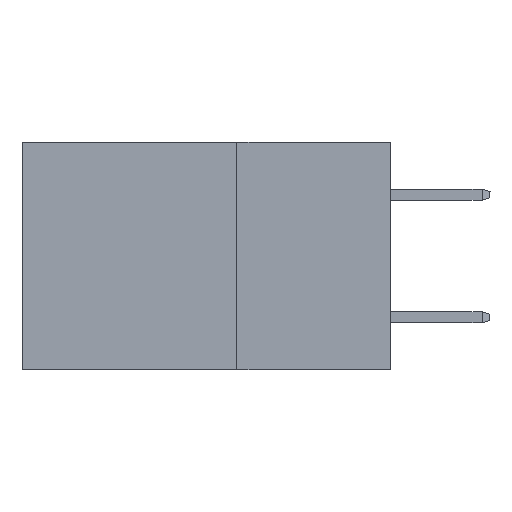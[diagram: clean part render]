
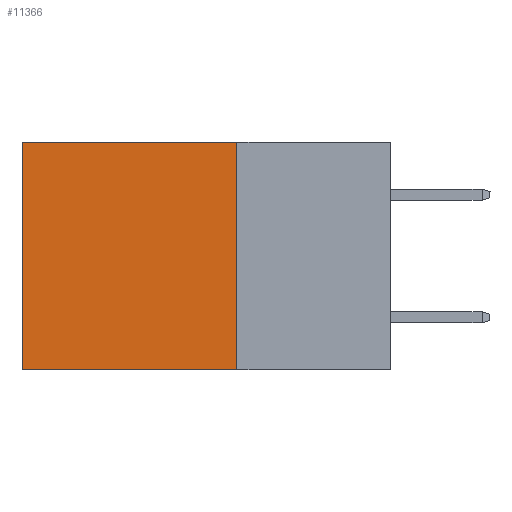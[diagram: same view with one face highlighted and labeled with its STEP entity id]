
A CAD part, left-side view. The second image highlights one B-rep face of the part: STEP entity #11366.
In plain terms, the highlighted planar face has unit normal (-1, 0, 0).
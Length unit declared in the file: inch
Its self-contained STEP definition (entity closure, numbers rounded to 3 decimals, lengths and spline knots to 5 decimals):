
#605 = CARTESIAN_POINT ( 'NONE',  ( 0.2875, 0.25, 0. ) ) ;
#1740 = VERTEX_POINT ( 'NONE', #13601 ) ;
#1962 = CARTESIAN_POINT ( 'NONE',  ( 0.2875, 0.25, 0. ) ) ;
#2853 = EDGE_CURVE ( 'NONE', #20786, #1740, #7967, .T. ) ;
#4057 = PLANE ( 'NONE',  #20959 ) ;
#6054 = ORIENTED_EDGE ( 'NONE', *, *, #20339, .T. ) ;
#6166 = VERTEX_POINT ( 'NONE', #6320 ) ;
#6305 = CARTESIAN_POINT ( 'NONE',  ( 0.2875, 0.25, 0. ) ) ;
#6320 = CARTESIAN_POINT ( 'NONE',  ( 0.2875, 0.25, -0.37 ) ) ;
#7039 = VECTOR ( 'NONE', #7184, 39.37008 ) ;
#7184 = DIRECTION ( 'NONE',  ( 0., 1., 0. ) ) ;
#7634 = DIRECTION ( 'NONE',  ( 1., 0., 0. ) ) ;
#7967 = LINE ( 'NONE', #13426, #21294 ) ;
#8365 = CARTESIAN_POINT ( 'NONE',  ( 0.2875, 0.6, 0. ) ) ;
#10256 = EDGE_CURVE ( 'NONE', #6166, #1740, #15493, .T. ) ;
#11265 = CARTESIAN_POINT ( 'NONE',  ( 0.2875, 0.25, -0.37 ) ) ;
#11366 = ADVANCED_FACE ( 'NONE', ( #20849 ), #4057, .F. ) ;
#11395 = VECTOR ( 'NONE', #18230, 39.37008 ) ;
#12250 = VERTEX_POINT ( 'NONE', #6305 ) ;
#12345 = ORIENTED_EDGE ( 'NONE', *, *, #10256, .F. ) ;
#13426 = CARTESIAN_POINT ( 'NONE',  ( 0.2875, 0.6, 0. ) ) ;
#13601 = CARTESIAN_POINT ( 'NONE',  ( 0.2875, 0.6, -0.37 ) ) ;
#15170 = ORIENTED_EDGE ( 'NONE', *, *, #2853, .T. ) ;
#15493 = LINE ( 'NONE', #11265, #11395 ) ;
#15971 = DIRECTION ( 'NONE',  ( 0., 0., -1. ) ) ;
#16050 = DIRECTION ( 'NONE',  ( 0., 0., -1. ) ) ;
#16476 = ORIENTED_EDGE ( 'NONE', *, *, #17909, .F. ) ;
#17909 = EDGE_CURVE ( 'NONE', #12250, #6166, #22527, .T. ) ;
#17998 = LINE ( 'NONE', #1962, #7039 ) ;
#18230 = DIRECTION ( 'NONE',  ( 0., 1., 0. ) ) ;
#19849 = DIRECTION ( 'NONE',  ( 0., 0., -1. ) ) ;
#20339 = EDGE_CURVE ( 'NONE', #12250, #20786, #17998, .T. ) ;
#20759 = EDGE_LOOP ( 'NONE', ( #15170, #12345, #16476, #6054 ) ) ;
#20786 = VERTEX_POINT ( 'NONE', #8365 ) ;
#20849 = FACE_OUTER_BOUND ( 'NONE', #20759, .T. ) ;
#20959 = AXIS2_PLACEMENT_3D ( 'NONE', #605, #7634, #19849 ) ;
#21182 = CARTESIAN_POINT ( 'NONE',  ( 0.2875, 0.25, 0. ) ) ;
#21294 = VECTOR ( 'NONE', #15971, 39.37008 ) ;
#22004 = VECTOR ( 'NONE', #16050, 39.37008 ) ;
#22527 = LINE ( 'NONE', #21182, #22004 ) ;
